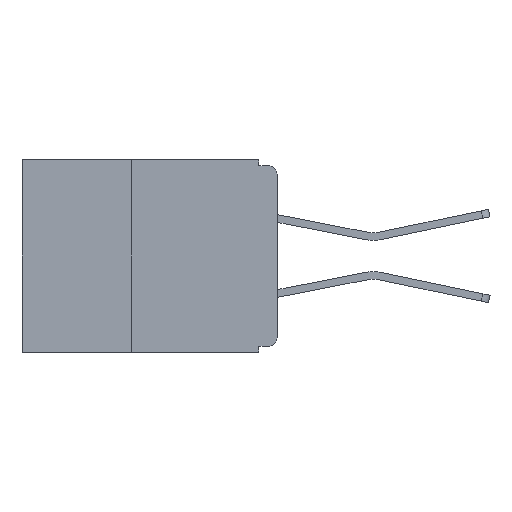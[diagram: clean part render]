
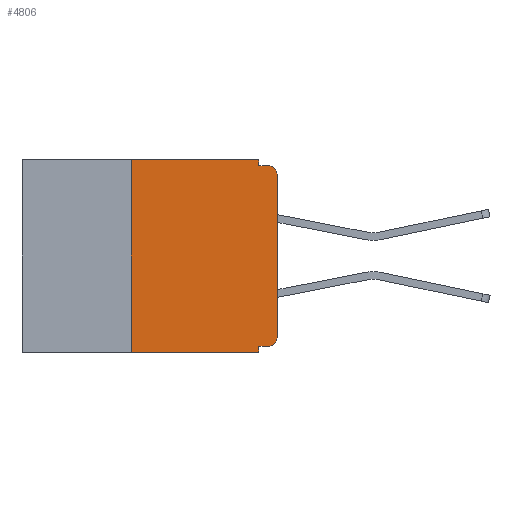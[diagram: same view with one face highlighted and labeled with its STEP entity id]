
A CAD part, left-side view. The second image highlights one B-rep face of the part: STEP entity #4806.
In plain terms, the highlighted planar face has unit normal (-1, 0, 0).
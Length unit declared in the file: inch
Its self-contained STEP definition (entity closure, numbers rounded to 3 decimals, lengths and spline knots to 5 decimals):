
#51 = EDGE_CURVE ( 'NONE', #12905, #16521, #6515, .T. ) ;
#656 = DIRECTION ( 'NONE',  ( 0., -1., 0. ) ) ;
#1376 = EDGE_CURVE ( 'NONE', #6599, #16521, #17932, .T. ) ;
#1483 = DIRECTION ( 'NONE',  ( 0., 0., -1. ) ) ;
#1502 = DIRECTION ( 'NONE',  ( -1., 0., 0. ) ) ;
#1516 = CARTESIAN_POINT ( 'NONE',  ( 0., 0.015, -0.305 ) ) ;
#1573 = AXIS2_PLACEMENT_3D ( 'NONE', #1516, #1502, #1483 ) ;
#2426 = CARTESIAN_POINT ( 'NONE',  ( 0., 0., -0.025 ) ) ;
#2474 = EDGE_CURVE ( 'NONE', #7007, #7172, #15782, .T. ) ;
#2586 = ORIENTED_EDGE ( 'NONE', *, *, #51, .T. ) ;
#2602 = VERTEX_POINT ( 'NONE', #13084 ) ;
#2707 = VECTOR ( 'NONE', #15567, 39.37008 ) ;
#3215 = EDGE_CURVE ( 'NONE', #10773, #7172, #10062, .T. ) ;
#3349 = VECTOR ( 'NONE', #5212, 39.37008 ) ;
#3507 = VECTOR ( 'NONE', #6439, 39.37008 ) ;
#3520 = ORIENTED_EDGE ( 'NONE', *, *, #4847, .F. ) ;
#3732 = ORIENTED_EDGE ( 'NONE', *, *, #15484, .F. ) ;
#3752 = ORIENTED_EDGE ( 'NONE', *, *, #8831, .T. ) ;
#3956 = EDGE_CURVE ( 'NONE', #2602, #4788, #10682, .T. ) ;
#4510 = CARTESIAN_POINT ( 'NONE',  ( 0., 0., -0.01 ) ) ;
#4788 = VERTEX_POINT ( 'NONE', #8523 ) ;
#4806 = ADVANCED_FACE ( 'NONE', ( #11983 ), #6971, .F. ) ;
#4847 = EDGE_CURVE ( 'NONE', #7007, #2602, #11105, .T. ) ;
#5184 = EDGE_LOOP ( 'NONE', ( #16882, #2586, #15851, #3732, #11466, #3520, #14990, #8473, #6528, #3752 ) ) ;
#5212 = DIRECTION ( 'NONE',  ( 0., 0., 1. ) ) ;
#5570 = CARTESIAN_POINT ( 'NONE',  ( 0., 0.25, -0.33 ) ) ;
#6072 = DIRECTION ( 'NONE',  ( 0., 0., -1. ) ) ;
#6439 = DIRECTION ( 'NONE',  ( 0., 0., 1. ) ) ;
#6465 = CARTESIAN_POINT ( 'NONE',  ( 0., 0., 0. ) ) ;
#6515 = CIRCLE ( 'NONE', #8578, 0.015 ) ;
#6528 = ORIENTED_EDGE ( 'NONE', *, *, #9374, .F. ) ;
#6594 = DIRECTION ( 'NONE',  ( -1., 0., 0. ) ) ;
#6599 = VERTEX_POINT ( 'NONE', #8163 ) ;
#6726 = CARTESIAN_POINT ( 'NONE',  ( 0., 0.031, -0.32 ) ) ;
#6853 = DIRECTION ( 'NONE',  ( 0., 0., -1. ) ) ;
#6872 = DIRECTION ( 'NONE',  ( 1., 0., 0. ) ) ;
#6971 = PLANE ( 'NONE',  #8296 ) ;
#7007 = VERTEX_POINT ( 'NONE', #17620 ) ;
#7160 = VECTOR ( 'NONE', #6072, 39.37008 ) ;
#7172 = VERTEX_POINT ( 'NONE', #16171 ) ;
#7175 = LINE ( 'NONE', #6465, #3507 ) ;
#7344 = VECTOR ( 'NONE', #656, 39.37008 ) ;
#7382 = CARTESIAN_POINT ( 'NONE',  ( 0., 0.437, 0. ) ) ;
#7782 = LINE ( 'NONE', #9458, #11420 ) ;
#8163 = CARTESIAN_POINT ( 'NONE',  ( 0., 0.031, -0.01 ) ) ;
#8296 = AXIS2_PLACEMENT_3D ( 'NONE', #7382, #6872, #6853 ) ;
#8315 = EDGE_CURVE ( 'NONE', #9773, #12905, #7175, .T. ) ;
#8473 = ORIENTED_EDGE ( 'NONE', *, *, #3215, .F. ) ;
#8523 = CARTESIAN_POINT ( 'NONE',  ( 0., 0.031, 0. ) ) ;
#8578 = AXIS2_PLACEMENT_3D ( 'NONE', #16913, #6594, #15145 ) ;
#8831 = EDGE_CURVE ( 'NONE', #13234, #9773, #12309, .T. ) ;
#9048 = DIRECTION ( 'NONE',  ( 0., 1., 0. ) ) ;
#9374 = EDGE_CURVE ( 'NONE', #13234, #10773, #7782, .T. ) ;
#9458 = CARTESIAN_POINT ( 'NONE',  ( 0., 0., -0.32 ) ) ;
#9773 = VERTEX_POINT ( 'NONE', #16932 ) ;
#9933 = LINE ( 'NONE', #14383, #7160 ) ;
#10062 = LINE ( 'NONE', #16458, #2707 ) ;
#10682 = LINE ( 'NONE', #12144, #13522 ) ;
#10773 = VERTEX_POINT ( 'NONE', #6726 ) ;
#11105 = LINE ( 'NONE', #5570, #3349 ) ;
#11174 = VECTOR ( 'NONE', #17954, 39.37008 ) ;
#11420 = VECTOR ( 'NONE', #9048, 39.37008 ) ;
#11466 = ORIENTED_EDGE ( 'NONE', *, *, #3956, .F. ) ;
#11797 = CARTESIAN_POINT ( 'NONE',  ( 0., 0.437, -0.33 ) ) ;
#11973 = DIRECTION ( 'NONE',  ( 0., -1., 0. ) ) ;
#11983 = FACE_OUTER_BOUND ( 'NONE', #5184, .T. ) ;
#12144 = CARTESIAN_POINT ( 'NONE',  ( 0., 0.437, 0. ) ) ;
#12309 = CIRCLE ( 'NONE', #1573, 0.015 ) ;
#12905 = VERTEX_POINT ( 'NONE', #2426 ) ;
#13084 = CARTESIAN_POINT ( 'NONE',  ( 0., 0.25, 0. ) ) ;
#13234 = VERTEX_POINT ( 'NONE', #15663 ) ;
#13522 = VECTOR ( 'NONE', #11973, 39.37008 ) ;
#14383 = CARTESIAN_POINT ( 'NONE',  ( 0., 0.031, 0. ) ) ;
#14990 = ORIENTED_EDGE ( 'NONE', *, *, #2474, .T. ) ;
#15145 = DIRECTION ( 'NONE',  ( 0., 0., -1. ) ) ;
#15332 = CARTESIAN_POINT ( 'NONE',  ( 0., 0.015, -0.01 ) ) ;
#15484 = EDGE_CURVE ( 'NONE', #4788, #6599, #9933, .T. ) ;
#15567 = DIRECTION ( 'NONE',  ( 0., 0., -1. ) ) ;
#15663 = CARTESIAN_POINT ( 'NONE',  ( 0., 0.015, -0.32 ) ) ;
#15782 = LINE ( 'NONE', #11797, #11174 ) ;
#15851 = ORIENTED_EDGE ( 'NONE', *, *, #1376, .F. ) ;
#16171 = CARTESIAN_POINT ( 'NONE',  ( 0., 0.031, -0.33 ) ) ;
#16458 = CARTESIAN_POINT ( 'NONE',  ( 0., 0.031, -0.33 ) ) ;
#16521 = VERTEX_POINT ( 'NONE', #15332 ) ;
#16882 = ORIENTED_EDGE ( 'NONE', *, *, #8315, .T. ) ;
#16913 = CARTESIAN_POINT ( 'NONE',  ( 0., 0.015, -0.025 ) ) ;
#16932 = CARTESIAN_POINT ( 'NONE',  ( 0., 0., -0.305 ) ) ;
#17620 = CARTESIAN_POINT ( 'NONE',  ( 0., 0.25, -0.33 ) ) ;
#17932 = LINE ( 'NONE', #4510, #7344 ) ;
#17954 = DIRECTION ( 'NONE',  ( 0., -1., 0. ) ) ;
